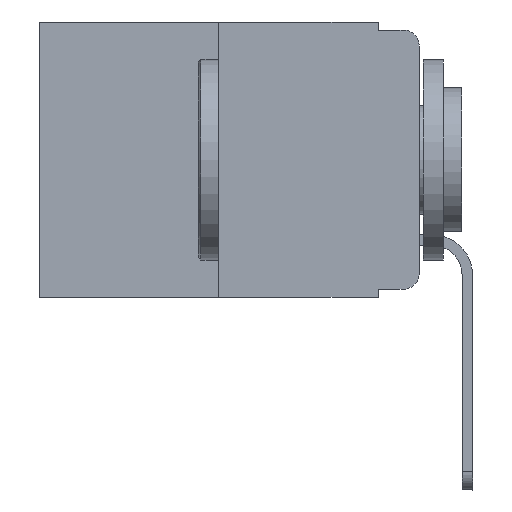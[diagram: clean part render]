
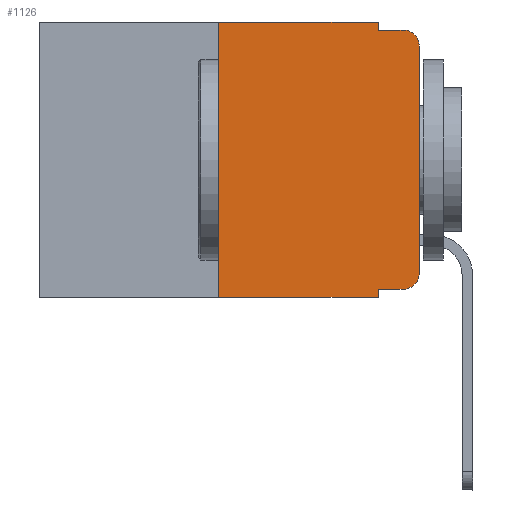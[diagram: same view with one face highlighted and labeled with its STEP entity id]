
A CAD part, left-side view. The second image highlights one B-rep face of the part: STEP entity #1126.
In plain terms, the highlighted planar face has unit normal (-1, 0, 0).
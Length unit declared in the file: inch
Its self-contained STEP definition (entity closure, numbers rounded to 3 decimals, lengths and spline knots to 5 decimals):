
#117 = AXIS2_PLACEMENT_3D ( 'NONE', #13713, #12966, #1501 ) ;
#301 = VERTEX_POINT ( 'NONE', #1861 ) ;
#608 = DIRECTION ( 'NONE',  ( 0., -1., 0. ) ) ;
#660 = DIRECTION ( 'NONE',  ( 0., 0., 1. ) ) ;
#1126 = ADVANCED_FACE ( 'NONE', ( #5592 ), #15550, .F. ) ;
#1290 = VERTEX_POINT ( 'NONE', #12159 ) ;
#1294 = LINE ( 'NONE', #12225, #2971 ) ;
#1308 = DIRECTION ( 'NONE',  ( 0., -1., 0. ) ) ;
#1355 = EDGE_CURVE ( 'NONE', #11411, #8559, #7667, .T. ) ;
#1501 = DIRECTION ( 'NONE',  ( 0., 0., -1. ) ) ;
#1861 = CARTESIAN_POINT ( 'NONE',  ( 0., 0.25, -0.343 ) ) ;
#2217 = LINE ( 'NONE', #12023, #14954 ) ;
#2536 = EDGE_CURVE ( 'NONE', #301, #13656, #2217, .T. ) ;
#2636 = DIRECTION ( 'NONE',  ( 0., 0., -1. ) ) ;
#2971 = VECTOR ( 'NONE', #11021, 39.37008 ) ;
#3040 = CARTESIAN_POINT ( 'NONE',  ( 0., 0.051, -0.343 ) ) ;
#3173 = EDGE_CURVE ( 'NONE', #11411, #13656, #3904, .T. ) ;
#3268 = LINE ( 'NONE', #14760, #5796 ) ;
#3314 = CARTESIAN_POINT ( 'NONE',  ( 0., 0.02, -0.01 ) ) ;
#3476 = DIRECTION ( 'NONE',  ( 0., 0., -1. ) ) ;
#3485 = EDGE_CURVE ( 'NONE', #8559, #4952, #8541, .T. ) ;
#3642 = DIRECTION ( 'NONE',  ( -1., 0., 0. ) ) ;
#3904 = LINE ( 'NONE', #15161, #4652 ) ;
#4101 = ORIENTED_EDGE ( 'NONE', *, *, #7307, .F. ) ;
#4147 = CARTESIAN_POINT ( 'NONE',  ( 0., 0.473, 0. ) ) ;
#4588 = DIRECTION ( 'NONE',  ( 0., -1., 0. ) ) ;
#4652 = VECTOR ( 'NONE', #8729, 39.37008 ) ;
#4827 = CARTESIAN_POINT ( 'NONE',  ( 0., 0., -0.03 ) ) ;
#4952 = VERTEX_POINT ( 'NONE', #15376 ) ;
#5247 = CARTESIAN_POINT ( 'NONE',  ( 0., 0.051, -0.333 ) ) ;
#5592 = FACE_OUTER_BOUND ( 'NONE', #14263, .T. ) ;
#5622 = ORIENTED_EDGE ( 'NONE', *, *, #9916, .F. ) ;
#5796 = VECTOR ( 'NONE', #6161, 39.37008 ) ;
#5808 = CARTESIAN_POINT ( 'NONE',  ( 0., 0., 0. ) ) ;
#5858 = ORIENTED_EDGE ( 'NONE', *, *, #3173, .F. ) ;
#6140 = CARTESIAN_POINT ( 'NONE',  ( 0., 0.02, -0.313 ) ) ;
#6161 = DIRECTION ( 'NONE',  ( 0., 0., -1. ) ) ;
#6194 = ORIENTED_EDGE ( 'NONE', *, *, #12149, .T. ) ;
#6702 = LINE ( 'NONE', #5808, #9177 ) ;
#6783 = LINE ( 'NONE', #8063, #13291 ) ;
#7057 = DIRECTION ( 'NONE',  ( 0., -1., 0. ) ) ;
#7307 = EDGE_CURVE ( 'NONE', #1290, #15142, #6783, .T. ) ;
#7311 = EDGE_CURVE ( 'NONE', #4952, #8700, #6702, .T. ) ;
#7533 = CARTESIAN_POINT ( 'NONE',  ( 0., 0.051, -0.333 ) ) ;
#7667 = LINE ( 'NONE', #5247, #7741 ) ;
#7700 = CARTESIAN_POINT ( 'NONE',  ( 0., 0.051, 0. ) ) ;
#7741 = VECTOR ( 'NONE', #1308, 39.37008 ) ;
#8032 = CARTESIAN_POINT ( 'NONE',  ( 0., 0.25, 0. ) ) ;
#8063 = CARTESIAN_POINT ( 'NONE',  ( 0., 0.051, -0.01 ) ) ;
#8379 = EDGE_CURVE ( 'NONE', #14027, #1290, #3268, .T. ) ;
#8541 = CIRCLE ( 'NONE', #13403, 0.02 ) ;
#8559 = VERTEX_POINT ( 'NONE', #11669 ) ;
#8667 = AXIS2_PLACEMENT_3D ( 'NONE', #11093, #13567, #2636 ) ;
#8700 = VERTEX_POINT ( 'NONE', #4827 ) ;
#8717 = EDGE_CURVE ( 'NONE', #301, #11155, #1294, .T. ) ;
#8729 = DIRECTION ( 'NONE',  ( 0., 0., -1. ) ) ;
#8831 = ORIENTED_EDGE ( 'NONE', *, *, #8379, .F. ) ;
#9177 = VECTOR ( 'NONE', #660, 39.37008 ) ;
#9916 = EDGE_CURVE ( 'NONE', #11155, #14027, #14271, .T. ) ;
#10695 = VECTOR ( 'NONE', #608, 39.37008 ) ;
#11021 = DIRECTION ( 'NONE',  ( 0., 0., 1. ) ) ;
#11093 = CARTESIAN_POINT ( 'NONE',  ( 0., 0.02, -0.03 ) ) ;
#11155 = VERTEX_POINT ( 'NONE', #8032 ) ;
#11411 = VERTEX_POINT ( 'NONE', #7533 ) ;
#11669 = CARTESIAN_POINT ( 'NONE',  ( 0., 0.02, -0.333 ) ) ;
#11748 = CIRCLE ( 'NONE', #8667, 0.02 ) ;
#12023 = CARTESIAN_POINT ( 'NONE',  ( 0., 0.473, -0.343 ) ) ;
#12149 = EDGE_CURVE ( 'NONE', #8700, #15142, #11748, .T. ) ;
#12159 = CARTESIAN_POINT ( 'NONE',  ( 0., 0.051, -0.01 ) ) ;
#12225 = CARTESIAN_POINT ( 'NONE',  ( 0., 0.25, 0. ) ) ;
#12966 = DIRECTION ( 'NONE',  ( 1., 0., 0. ) ) ;
#13075 = ORIENTED_EDGE ( 'NONE', *, *, #3485, .T. ) ;
#13291 = VECTOR ( 'NONE', #4588, 39.37008 ) ;
#13403 = AXIS2_PLACEMENT_3D ( 'NONE', #6140, #3642, #3476 ) ;
#13567 = DIRECTION ( 'NONE',  ( -1., 0., 0. ) ) ;
#13656 = VERTEX_POINT ( 'NONE', #3040 ) ;
#13692 = ORIENTED_EDGE ( 'NONE', *, *, #2536, .T. ) ;
#13713 = CARTESIAN_POINT ( 'NONE',  ( 0., 0.473, 0. ) ) ;
#14027 = VERTEX_POINT ( 'NONE', #7700 ) ;
#14263 = EDGE_LOOP ( 'NONE', ( #14455, #6194, #4101, #8831, #5622, #15526, #13692, #5858, #15713, #13075 ) ) ;
#14271 = LINE ( 'NONE', #4147, #10695 ) ;
#14455 = ORIENTED_EDGE ( 'NONE', *, *, #7311, .T. ) ;
#14760 = CARTESIAN_POINT ( 'NONE',  ( 0., 0.051, 0. ) ) ;
#14954 = VECTOR ( 'NONE', #7057, 39.37008 ) ;
#15142 = VERTEX_POINT ( 'NONE', #3314 ) ;
#15161 = CARTESIAN_POINT ( 'NONE',  ( 0., 0.051, 0. ) ) ;
#15376 = CARTESIAN_POINT ( 'NONE',  ( 0., 0., -0.313 ) ) ;
#15526 = ORIENTED_EDGE ( 'NONE', *, *, #8717, .F. ) ;
#15550 = PLANE ( 'NONE',  #117 ) ;
#15713 = ORIENTED_EDGE ( 'NONE', *, *, #1355, .T. ) ;
